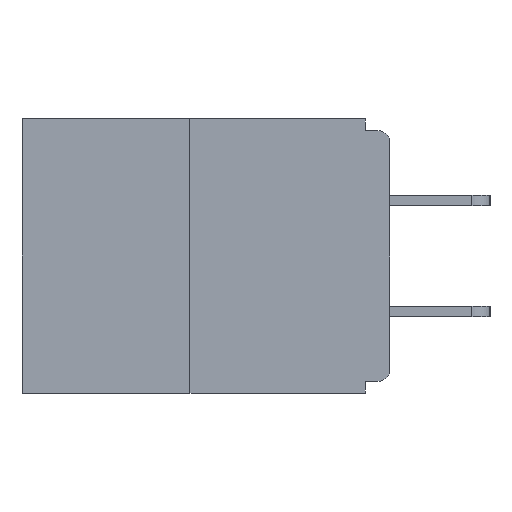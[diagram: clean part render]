
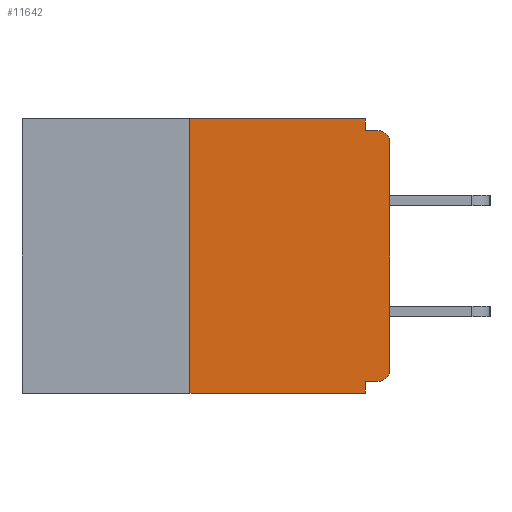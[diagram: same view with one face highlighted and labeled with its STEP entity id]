
A CAD part, left-side view. The second image highlights one B-rep face of the part: STEP entity #11642.
In plain terms, the highlighted planar face has unit normal (-1, 0, 0).
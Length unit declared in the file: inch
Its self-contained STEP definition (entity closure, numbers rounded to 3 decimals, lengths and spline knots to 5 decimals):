
#264 = CARTESIAN_POINT ( 'NONE',  ( 0., 0., 0. ) ) ;
#296 = DIRECTION ( 'NONE',  ( -1., 0., 0. ) ) ;
#514 = EDGE_CURVE ( 'NONE', #8615, #18993, #20384, .T. ) ;
#776 = VERTEX_POINT ( 'NONE', #15321 ) ;
#994 = ORIENTED_EDGE ( 'NONE', *, *, #514, .F. ) ;
#1460 = PLANE ( 'NONE',  #15372 ) ;
#1942 = ORIENTED_EDGE ( 'NONE', *, *, #14509, .F. ) ;
#2114 = VERTEX_POINT ( 'NONE', #17456 ) ;
#2264 = VECTOR ( 'NONE', #10003, 39.37008 ) ;
#2327 = VERTEX_POINT ( 'NONE', #10380 ) ;
#2701 = LINE ( 'NONE', #6206, #5048 ) ;
#2966 = DIRECTION ( 'NONE',  ( 1., 0., 0. ) ) ;
#3109 = CARTESIAN_POINT ( 'NONE',  ( 0., 0.46, 0. ) ) ;
#3858 = VERTEX_POINT ( 'NONE', #4028 ) ;
#3934 = DIRECTION ( 'NONE',  ( 0., 1., 0. ) ) ;
#4028 = CARTESIAN_POINT ( 'NONE',  ( 0., 0.25, -0.343 ) ) ;
#4265 = FACE_OUTER_BOUND ( 'NONE', #10354, .T. ) ;
#4377 = CARTESIAN_POINT ( 'NONE',  ( 0., 0.015, -0.313 ) ) ;
#4785 = DIRECTION ( 'NONE',  ( 0., 0., -1. ) ) ;
#5048 = VECTOR ( 'NONE', #16085, 39.37008 ) ;
#5272 = ORIENTED_EDGE ( 'NONE', *, *, #5620, .F. ) ;
#5620 = EDGE_CURVE ( 'NONE', #18904, #8615, #7717, .T. ) ;
#6206 = CARTESIAN_POINT ( 'NONE',  ( 0., 0.031, -0.343 ) ) ;
#6463 = CIRCLE ( 'NONE', #12339, 0.015 ) ;
#6476 = LINE ( 'NONE', #6515, #6749 ) ;
#6515 = CARTESIAN_POINT ( 'NONE',  ( 0., 0., -0.015 ) ) ;
#6744 = VERTEX_POINT ( 'NONE', #20059 ) ;
#6749 = VECTOR ( 'NONE', #19696, 39.37008 ) ;
#7090 = CARTESIAN_POINT ( 'NONE',  ( 0., 0., -0.328 ) ) ;
#7169 = LINE ( 'NONE', #13428, #2264 ) ;
#7717 = LINE ( 'NONE', #15040, #20375 ) ;
#7724 = DIRECTION ( 'NONE',  ( 0., 0., -1. ) ) ;
#7979 = ORIENTED_EDGE ( 'NONE', *, *, #15226, .T. ) ;
#8234 = VECTOR ( 'NONE', #10235, 39.37008 ) ;
#8615 = VERTEX_POINT ( 'NONE', #11175 ) ;
#9352 = ORIENTED_EDGE ( 'NONE', *, *, #14008, .F. ) ;
#9525 = ORIENTED_EDGE ( 'NONE', *, *, #20550, .T. ) ;
#10003 = DIRECTION ( 'NONE',  ( 0., -1., 0. ) ) ;
#10028 = EDGE_CURVE ( 'NONE', #11874, #6744, #19398, .T. ) ;
#10235 = DIRECTION ( 'NONE',  ( 0., 0., 1. ) ) ;
#10287 = CIRCLE ( 'NONE', #21187, 0.015 ) ;
#10354 = EDGE_LOOP ( 'NONE', ( #5272, #9352, #7979, #13543, #1942, #9525, #14038, #13973, #19329, #994 ) ) ;
#10380 = CARTESIAN_POINT ( 'NONE',  ( 0., 0.031, -0.328 ) ) ;
#10781 = LINE ( 'NONE', #7090, #13654 ) ;
#11175 = CARTESIAN_POINT ( 'NONE',  ( 0., 0.031, 0. ) ) ;
#11508 = EDGE_CURVE ( 'NONE', #2327, #776, #2701, .T. ) ;
#11618 = DIRECTION ( 'NONE',  ( 0., 0., 1. ) ) ;
#11642 = ADVANCED_FACE ( 'NONE', ( #4265 ), #1460, .F. ) ;
#11874 = VERTEX_POINT ( 'NONE', #17785 ) ;
#12339 = AXIS2_PLACEMENT_3D ( 'NONE', #13681, #296, #18432 ) ;
#12865 = CARTESIAN_POINT ( 'NONE',  ( 0., 0.25, 0. ) ) ;
#13428 = CARTESIAN_POINT ( 'NONE',  ( 0., 0.46, -0.343 ) ) ;
#13543 = ORIENTED_EDGE ( 'NONE', *, *, #11508, .F. ) ;
#13651 = CARTESIAN_POINT ( 'NONE',  ( 0., 0.031, -0.015 ) ) ;
#13654 = VECTOR ( 'NONE', #3934, 39.37008 ) ;
#13681 = CARTESIAN_POINT ( 'NONE',  ( 0., 0.015, -0.03 ) ) ;
#13973 = ORIENTED_EDGE ( 'NONE', *, *, #20302, .T. ) ;
#14008 = EDGE_CURVE ( 'NONE', #3858, #18904, #18819, .T. ) ;
#14038 = ORIENTED_EDGE ( 'NONE', *, *, #10028, .T. ) ;
#14509 = EDGE_CURVE ( 'NONE', #17698, #2327, #10781, .T. ) ;
#15040 = CARTESIAN_POINT ( 'NONE',  ( 0., 0.46, 0. ) ) ;
#15226 = EDGE_CURVE ( 'NONE', #3858, #776, #7169, .T. ) ;
#15321 = CARTESIAN_POINT ( 'NONE',  ( 0., 0.031, -0.343 ) ) ;
#15372 = AXIS2_PLACEMENT_3D ( 'NONE', #3109, #2966, #4785 ) ;
#15694 = DIRECTION ( 'NONE',  ( 0., -1., 0. ) ) ;
#16014 = VECTOR ( 'NONE', #20809, 39.37008 ) ;
#16085 = DIRECTION ( 'NONE',  ( 0., 0., -1. ) ) ;
#16852 = VECTOR ( 'NONE', #11618, 39.37008 ) ;
#16876 = CARTESIAN_POINT ( 'NONE',  ( 0., 0.015, -0.328 ) ) ;
#17456 = CARTESIAN_POINT ( 'NONE',  ( 0., 0.015, -0.015 ) ) ;
#17698 = VERTEX_POINT ( 'NONE', #16876 ) ;
#17785 = CARTESIAN_POINT ( 'NONE',  ( 0., 0., -0.313 ) ) ;
#18432 = DIRECTION ( 'NONE',  ( 0., 0., -1. ) ) ;
#18819 = LINE ( 'NONE', #20120, #8234 ) ;
#18870 = EDGE_CURVE ( 'NONE', #18993, #2114, #6476, .T. ) ;
#18904 = VERTEX_POINT ( 'NONE', #12865 ) ;
#18993 = VERTEX_POINT ( 'NONE', #13651 ) ;
#19055 = DIRECTION ( 'NONE',  ( -1., 0., 0. ) ) ;
#19329 = ORIENTED_EDGE ( 'NONE', *, *, #18870, .F. ) ;
#19398 = LINE ( 'NONE', #264, #16852 ) ;
#19696 = DIRECTION ( 'NONE',  ( 0., -1., 0. ) ) ;
#20059 = CARTESIAN_POINT ( 'NONE',  ( 0., 0., -0.03 ) ) ;
#20120 = CARTESIAN_POINT ( 'NONE',  ( 0., 0.25, 0. ) ) ;
#20302 = EDGE_CURVE ( 'NONE', #6744, #2114, #6463, .T. ) ;
#20375 = VECTOR ( 'NONE', #15694, 39.37008 ) ;
#20384 = LINE ( 'NONE', #20740, #16014 ) ;
#20550 = EDGE_CURVE ( 'NONE', #17698, #11874, #10287, .T. ) ;
#20740 = CARTESIAN_POINT ( 'NONE',  ( 0., 0.031, 0. ) ) ;
#20809 = DIRECTION ( 'NONE',  ( 0., 0., -1. ) ) ;
#21187 = AXIS2_PLACEMENT_3D ( 'NONE', #4377, #19055, #7724 ) ;
